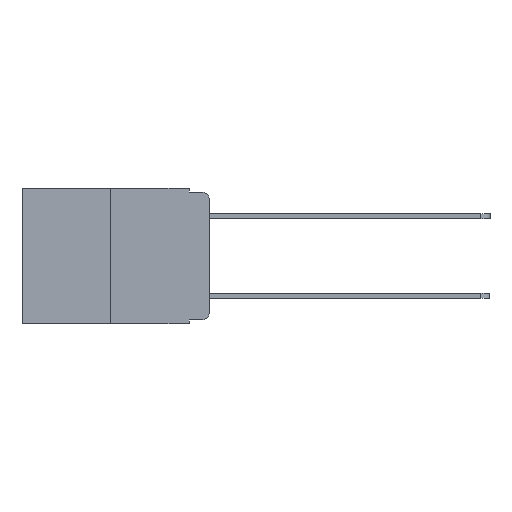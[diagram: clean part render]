
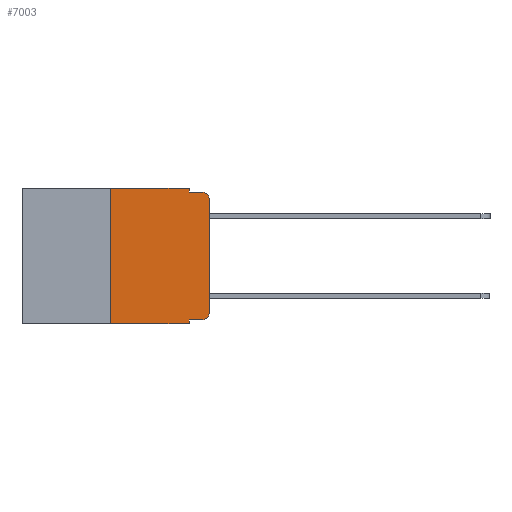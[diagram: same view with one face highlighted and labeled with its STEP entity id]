
A CAD part, left-side view. The second image highlights one B-rep face of the part: STEP entity #7003.
In plain terms, the highlighted planar face has unit normal (-1, 0, 0).
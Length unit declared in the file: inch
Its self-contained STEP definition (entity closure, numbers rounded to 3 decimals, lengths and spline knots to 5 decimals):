
#102 = EDGE_CURVE ( 'NONE', #6361, #2091, #10950, .T. ) ;
#110 = DIRECTION ( 'NONE',  ( 0., 0., -1. ) ) ;
#147 = CIRCLE ( 'NONE', #8288, 0.02 ) ;
#267 = CARTESIAN_POINT ( 'NONE',  ( 0., 0.051, -0.333 ) ) ;
#291 = VERTEX_POINT ( 'NONE', #10465 ) ;
#342 = EDGE_CURVE ( 'NONE', #10265, #2091, #10800, .T. ) ;
#504 = ORIENTED_EDGE ( 'NONE', *, *, #8712, .T. ) ;
#541 = EDGE_CURVE ( 'NONE', #9006, #5356, #1350, .T. ) ;
#615 = ORIENTED_EDGE ( 'NONE', *, *, #541, .T. ) ;
#680 = DIRECTION ( 'NONE',  ( 0., -1., 0. ) ) ;
#826 = CARTESIAN_POINT ( 'NONE',  ( 0., 0., 0. ) ) ;
#1146 = VERTEX_POINT ( 'NONE', #10409 ) ;
#1159 = CARTESIAN_POINT ( 'NONE',  ( 0., 0.473, 0. ) ) ;
#1165 = PLANE ( 'NONE',  #2450 ) ;
#1350 = LINE ( 'NONE', #5949, #3539 ) ;
#1371 = VECTOR ( 'NONE', #7354, 39.37008 ) ;
#1506 = ORIENTED_EDGE ( 'NONE', *, *, #9617, .F. ) ;
#1528 = AXIS2_PLACEMENT_3D ( 'NONE', #11362, #9823, #11309 ) ;
#1553 = VECTOR ( 'NONE', #8859, 39.37008 ) ;
#2020 = VERTEX_POINT ( 'NONE', #6770 ) ;
#2091 = VERTEX_POINT ( 'NONE', #8774 ) ;
#2450 = AXIS2_PLACEMENT_3D ( 'NONE', #3950, #9609, #4032 ) ;
#2519 = VERTEX_POINT ( 'NONE', #10622 ) ;
#2596 = CARTESIAN_POINT ( 'NONE',  ( 0., 0.25, 0. ) ) ;
#2838 = DIRECTION ( 'NONE',  ( -1., 0., 0. ) ) ;
#3127 = CARTESIAN_POINT ( 'NONE',  ( 0., 0.25, 0. ) ) ;
#3208 = ORIENTED_EDGE ( 'NONE', *, *, #11275, .T. ) ;
#3248 = CARTESIAN_POINT ( 'NONE',  ( 0., 0.473, -0.343 ) ) ;
#3531 = ORIENTED_EDGE ( 'NONE', *, *, #6109, .F. ) ;
#3539 = VECTOR ( 'NONE', #680, 39.37008 ) ;
#3733 = ORIENTED_EDGE ( 'NONE', *, *, #342, .T. ) ;
#3950 = CARTESIAN_POINT ( 'NONE',  ( 0., 0.473, 0. ) ) ;
#4032 = DIRECTION ( 'NONE',  ( 0., 0., -1. ) ) ;
#5045 = CARTESIAN_POINT ( 'NONE',  ( 0., 0.051, -0.01 ) ) ;
#5258 = EDGE_CURVE ( 'NONE', #9006, #2020, #10344, .T. ) ;
#5272 = FACE_OUTER_BOUND ( 'NONE', #5620, .T. ) ;
#5293 = VECTOR ( 'NONE', #8170, 39.37008 ) ;
#5356 = VERTEX_POINT ( 'NONE', #10284 ) ;
#5620 = EDGE_LOOP ( 'NONE', ( #504, #3733, #8406, #6951, #1506, #3531, #6269, #7499, #615, #3208 ) ) ;
#5740 = CARTESIAN_POINT ( 'NONE',  ( 0., 0.051, 0. ) ) ;
#5854 = CARTESIAN_POINT ( 'NONE',  ( 0., 0.051, -0.01 ) ) ;
#5949 = CARTESIAN_POINT ( 'NONE',  ( 0., 0.051, -0.333 ) ) ;
#6109 = EDGE_CURVE ( 'NONE', #2519, #8439, #10196, .T. ) ;
#6269 = ORIENTED_EDGE ( 'NONE', *, *, #7631, .T. ) ;
#6361 = VERTEX_POINT ( 'NONE', #5854 ) ;
#6523 = LINE ( 'NONE', #5740, #9270 ) ;
#6533 = LINE ( 'NONE', #3248, #1553 ) ;
#6766 = DIRECTION ( 'NONE',  ( 0., -1., 0. ) ) ;
#6770 = CARTESIAN_POINT ( 'NONE',  ( 0., 0.051, -0.343 ) ) ;
#6792 = LINE ( 'NONE', #1159, #11379 ) ;
#6951 = ORIENTED_EDGE ( 'NONE', *, *, #8026, .F. ) ;
#7003 = ADVANCED_FACE ( 'NONE', ( #5272 ), #1165, .F. ) ;
#7320 = VECTOR ( 'NONE', #11960, 39.37008 ) ;
#7354 = DIRECTION ( 'NONE',  ( 0., 0., 1. ) ) ;
#7364 = DIRECTION ( 'NONE',  ( 0., -1., 0. ) ) ;
#7499 = ORIENTED_EDGE ( 'NONE', *, *, #5258, .F. ) ;
#7631 = EDGE_CURVE ( 'NONE', #2519, #2020, #6533, .T. ) ;
#8026 = EDGE_CURVE ( 'NONE', #1146, #6361, #6523, .T. ) ;
#8170 = DIRECTION ( 'NONE',  ( 0., 0., 1. ) ) ;
#8288 = AXIS2_PLACEMENT_3D ( 'NONE', #8453, #2838, #9379 ) ;
#8406 = ORIENTED_EDGE ( 'NONE', *, *, #102, .F. ) ;
#8439 = VERTEX_POINT ( 'NONE', #3127 ) ;
#8453 = CARTESIAN_POINT ( 'NONE',  ( 0., 0.02, -0.313 ) ) ;
#8523 = VECTOR ( 'NONE', #7364, 39.37008 ) ;
#8712 = EDGE_CURVE ( 'NONE', #291, #10265, #11245, .T. ) ;
#8774 = CARTESIAN_POINT ( 'NONE',  ( 0., 0.02, -0.01 ) ) ;
#8859 = DIRECTION ( 'NONE',  ( 0., -1., 0. ) ) ;
#9006 = VERTEX_POINT ( 'NONE', #267 ) ;
#9270 = VECTOR ( 'NONE', #110, 39.37008 ) ;
#9379 = DIRECTION ( 'NONE',  ( 0., 0., -1. ) ) ;
#9609 = DIRECTION ( 'NONE',  ( 1., 0., 0. ) ) ;
#9617 = EDGE_CURVE ( 'NONE', #8439, #1146, #6792, .T. ) ;
#9823 = DIRECTION ( 'NONE',  ( -1., 0., 0. ) ) ;
#10134 = CARTESIAN_POINT ( 'NONE',  ( 0., 0.051, 0. ) ) ;
#10196 = LINE ( 'NONE', #2596, #5293 ) ;
#10265 = VERTEX_POINT ( 'NONE', #10539 ) ;
#10284 = CARTESIAN_POINT ( 'NONE',  ( 0., 0.02, -0.333 ) ) ;
#10344 = LINE ( 'NONE', #10134, #7320 ) ;
#10409 = CARTESIAN_POINT ( 'NONE',  ( 0., 0.051, 0. ) ) ;
#10465 = CARTESIAN_POINT ( 'NONE',  ( 0., 0., -0.313 ) ) ;
#10539 = CARTESIAN_POINT ( 'NONE',  ( 0., 0., -0.03 ) ) ;
#10622 = CARTESIAN_POINT ( 'NONE',  ( 0., 0.25, -0.343 ) ) ;
#10800 = CIRCLE ( 'NONE', #1528, 0.02 ) ;
#10950 = LINE ( 'NONE', #5045, #8523 ) ;
#11245 = LINE ( 'NONE', #826, #1371 ) ;
#11275 = EDGE_CURVE ( 'NONE', #5356, #291, #147, .T. ) ;
#11309 = DIRECTION ( 'NONE',  ( 0., 0., -1. ) ) ;
#11362 = CARTESIAN_POINT ( 'NONE',  ( 0., 0.02, -0.03 ) ) ;
#11379 = VECTOR ( 'NONE', #6766, 39.37008 ) ;
#11960 = DIRECTION ( 'NONE',  ( 0., 0., -1. ) ) ;
